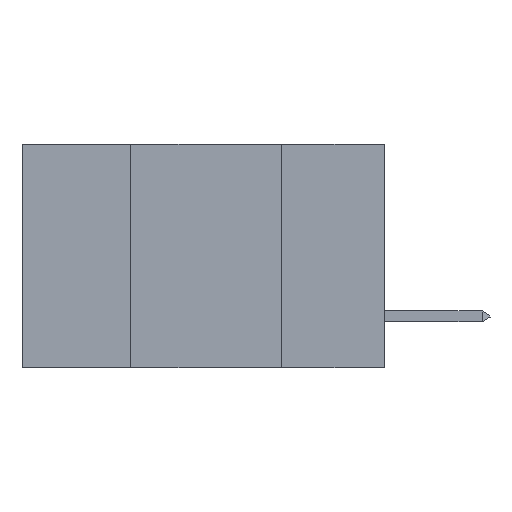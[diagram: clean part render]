
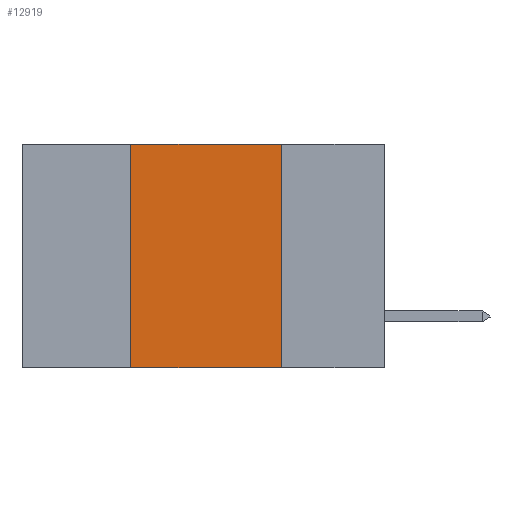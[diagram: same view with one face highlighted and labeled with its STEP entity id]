
A CAD part, left-side view. The second image highlights one B-rep face of the part: STEP entity #12919.
In plain terms, the highlighted planar face has unit normal (-1, 0, 0).
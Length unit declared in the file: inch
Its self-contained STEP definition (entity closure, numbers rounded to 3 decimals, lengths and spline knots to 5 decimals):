
#1219 = LINE ( 'NONE', #30953, #22604 ) ;
#5580 = VERTEX_POINT ( 'NONE', #16153 ) ;
#7107 = ORIENTED_EDGE ( 'NONE', *, *, #20736, .F. ) ;
#9071 = AXIS2_PLACEMENT_3D ( 'NONE', #40328, #33779, #19866 ) ;
#9506 = CARTESIAN_POINT ( 'NONE',  ( 0., 0.17, 0. ) ) ;
#9855 = CARTESIAN_POINT ( 'NONE',  ( 0., 0.6, 0. ) ) ;
#12919 = ADVANCED_FACE ( 'NONE', ( #23552 ), #33926, .F. ) ;
#15168 = DIRECTION ( 'NONE',  ( 0., -1., 0. ) ) ;
#16153 = CARTESIAN_POINT ( 'NONE',  ( 0., 0.42, -0.37 ) ) ;
#16658 = DIRECTION ( 'NONE',  ( 0., -1., 0. ) ) ;
#19866 = DIRECTION ( 'NONE',  ( 0., 0., -1. ) ) ;
#20736 = EDGE_CURVE ( 'NONE', #5580, #21028, #22849, .T. ) ;
#21028 = VERTEX_POINT ( 'NONE', #43145 ) ;
#22604 = VECTOR ( 'NONE', #33919, 39.37008 ) ;
#22849 = LINE ( 'NONE', #35871, #34006 ) ;
#23552 = FACE_OUTER_BOUND ( 'NONE', #42622, .T. ) ;
#24990 = VERTEX_POINT ( 'NONE', #32990 ) ;
#27703 = LINE ( 'NONE', #9855, #28815 ) ;
#28781 = EDGE_CURVE ( 'NONE', #21028, #37943, #27703, .T. ) ;
#28815 = VECTOR ( 'NONE', #16658, 39.37008 ) ;
#29477 = ORIENTED_EDGE ( 'NONE', *, *, #28781, .F. ) ;
#30953 = CARTESIAN_POINT ( 'NONE',  ( 0., 0.17, 0. ) ) ;
#32221 = EDGE_CURVE ( 'NONE', #37943, #24990, #1219, .T. ) ;
#32990 = CARTESIAN_POINT ( 'NONE',  ( 0., 0.17, -0.37 ) ) ;
#33779 = DIRECTION ( 'NONE',  ( 1., 0., 0. ) ) ;
#33919 = DIRECTION ( 'NONE',  ( 0., 0., -1. ) ) ;
#33926 = PLANE ( 'NONE',  #9071 ) ;
#34006 = VECTOR ( 'NONE', #42595, 39.37008 ) ;
#35103 = VECTOR ( 'NONE', #15168, 39.37008 ) ;
#35570 = CARTESIAN_POINT ( 'NONE',  ( 0., 0.6, -0.37 ) ) ;
#35871 = CARTESIAN_POINT ( 'NONE',  ( 0., 0.42, 0. ) ) ;
#36381 = ORIENTED_EDGE ( 'NONE', *, *, #32221, .F. ) ;
#37851 = ORIENTED_EDGE ( 'NONE', *, *, #41447, .T. ) ;
#37943 = VERTEX_POINT ( 'NONE', #9506 ) ;
#40328 = CARTESIAN_POINT ( 'NONE',  ( 0., 0.6, 0. ) ) ;
#40499 = LINE ( 'NONE', #35570, #35103 ) ;
#41447 = EDGE_CURVE ( 'NONE', #5580, #24990, #40499, .T. ) ;
#42595 = DIRECTION ( 'NONE',  ( 0., 0., 1. ) ) ;
#42622 = EDGE_LOOP ( 'NONE', ( #36381, #29477, #7107, #37851 ) ) ;
#43145 = CARTESIAN_POINT ( 'NONE',  ( 0., 0.42, 0. ) ) ;
